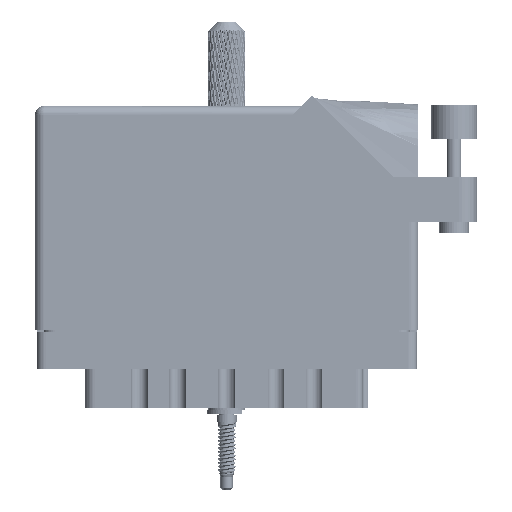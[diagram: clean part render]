
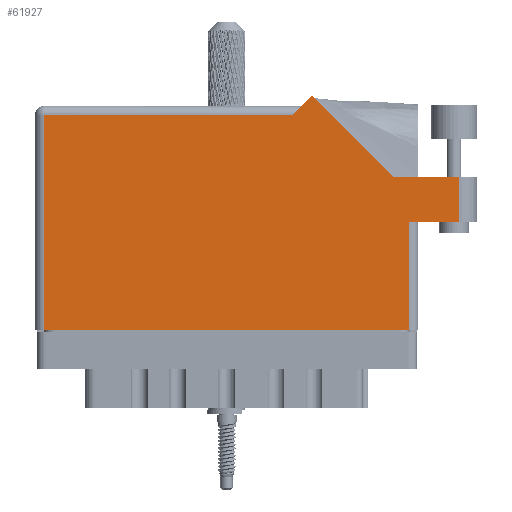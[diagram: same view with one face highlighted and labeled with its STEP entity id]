
A CAD part, front view. The second image highlights one B-rep face of the part: STEP entity #61927.
In plain terms, the highlighted face is planar.
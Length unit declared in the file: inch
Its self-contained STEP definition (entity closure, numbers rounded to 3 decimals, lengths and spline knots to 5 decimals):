
#148 = DIRECTION ( 'NONE',  ( -0.707, -0.707, 0. ) ) ;
#221 = CARTESIAN_POINT ( 'NONE',  ( 2.612, 0.737, 0. ) ) ;
#1091 = VECTOR ( 'NONE', #113292, 39.37008 ) ;
#3236 = ORIENTED_EDGE ( 'NONE', *, *, #10698, .T. ) ;
#4118 = CARTESIAN_POINT ( 'NONE',  ( 3.012, 1.044, 0. ) ) ;
#5088 = PLANE ( 'NONE',  #23254 ) ;
#5506 = CARTESIAN_POINT ( 'NONE',  ( 2.55, 0.737, 0. ) ) ;
#5569 = ORIENTED_EDGE ( 'NONE', *, *, #105520, .T. ) ;
#5610 = VECTOR ( 'NONE', #78746, 39.37008 ) ;
#6254 = ORIENTED_EDGE ( 'NONE', *, *, #28979, .T. ) ;
#9089 = ORIENTED_EDGE ( 'NONE', *, *, #114482, .T. ) ;
#10331 = VERTEX_POINT ( 'NONE', #107970 ) ;
#10432 = EDGE_CURVE ( 'NONE', #11539, #47254, #103604, .T. ) ;
#10698 = EDGE_CURVE ( 'NONE', #10331, #19697, #19981, .T. ) ;
#11539 = VERTEX_POINT ( 'NONE', #89694 ) ;
#16987 = CARTESIAN_POINT ( 'NONE',  ( 0.062, 1.468, 0. ) ) ;
#18177 = CARTESIAN_POINT ( 'NONE',  ( 1.88971, 1.60071, 0. ) ) ;
#19497 = CARTESIAN_POINT ( 'NONE',  ( 2.887, 1.044, 0. ) ) ;
#19697 = VERTEX_POINT ( 'NONE', #18177 ) ;
#19981 = LINE ( 'NONE', #33918, #57261 ) ;
#20785 = DIRECTION ( 'NONE',  ( 0., 1., 0. ) ) ;
#22708 = ORIENTED_EDGE ( 'NONE', *, *, #89235, .T. ) ;
#23254 = AXIS2_PLACEMENT_3D ( 'NONE', #51756, #69391, #118235 ) ;
#23885 = DIRECTION ( 'NONE',  ( -0.707, 0.707, 0. ) ) ;
#24387 = LINE ( 'NONE', #19497, #94914 ) ;
#24979 = ORIENTED_EDGE ( 'NONE', *, *, #115532, .T. ) ;
#25235 = VECTOR ( 'NONE', #41945, 39.37008 ) ;
#28131 = EDGE_LOOP ( 'NONE', ( #24979, #9089, #22708, #3236, #73229, #102067, #106604, #6254, #5569 ) ) ;
#28979 = EDGE_CURVE ( 'NONE', #78155, #74964, #81233, .T. ) ;
#33918 = CARTESIAN_POINT ( 'NONE',  ( 2.44642, 1.044, 0. ) ) ;
#35378 = DIRECTION ( 'NONE',  ( 0., -1., 0. ) ) ;
#35603 = CARTESIAN_POINT ( 'NONE',  ( 1.819, 1.53, 0. ) ) ;
#41945 = DIRECTION ( 'NONE',  ( -1., 0., 0. ) ) ;
#43129 = VERTEX_POINT ( 'NONE', #89583 ) ;
#47254 = VERTEX_POINT ( 'NONE', #16987 ) ;
#47324 = CARTESIAN_POINT ( 'NONE',  ( 2.55, 0.737, 0. ) ) ;
#49379 = CARTESIAN_POINT ( 'NONE',  ( 0., 1.468, 0. ) ) ;
#49809 = CARTESIAN_POINT ( 'NONE',  ( 0., 0., 0. ) ) ;
#51756 = CARTESIAN_POINT ( 'NONE',  ( 0., 1.53, 0. ) ) ;
#54498 = VECTOR ( 'NONE', #35378, 39.37008 ) ;
#56486 = LINE ( 'NONE', #47324, #67952 ) ;
#57261 = VECTOR ( 'NONE', #23885, 39.37008 ) ;
#59903 = VERTEX_POINT ( 'NONE', #5506 ) ;
#61114 = LINE ( 'NONE', #35603, #95768 ) ;
#61927 = ADVANCED_FACE ( 'NONE', ( #89214 ), #5088, .F. ) ;
#67807 = DIRECTION ( 'NONE',  ( 1., 0., 0. ) ) ;
#67952 = VECTOR ( 'NONE', #20785, 39.37008 ) ;
#69391 = DIRECTION ( 'NONE',  ( 0., 0., -1. ) ) ;
#70201 = EDGE_CURVE ( 'NONE', #47254, #78155, #79018, .T. ) ;
#73229 = ORIENTED_EDGE ( 'NONE', *, *, #113468, .T. ) ;
#74438 = LINE ( 'NONE', #221, #1091 ) ;
#74964 = VERTEX_POINT ( 'NONE', #119084 ) ;
#78155 = VERTEX_POINT ( 'NONE', #96973 ) ;
#78746 = DIRECTION ( 'NONE',  ( -1., 0., 0. ) ) ;
#79018 = LINE ( 'NONE', #99855, #54498 ) ;
#81233 = LINE ( 'NONE', #49809, #91260 ) ;
#87028 = LINE ( 'NONE', #4118, #25235 ) ;
#89214 = FACE_OUTER_BOUND ( 'NONE', #28131, .T. ) ;
#89235 = EDGE_CURVE ( 'NONE', #104139, #10331, #87028, .T. ) ;
#89583 = CARTESIAN_POINT ( 'NONE',  ( 2.887, 0.737, 0. ) ) ;
#89694 = CARTESIAN_POINT ( 'NONE',  ( 1.757, 1.468, 0. ) ) ;
#91260 = VECTOR ( 'NONE', #67807, 39.37008 ) ;
#94914 = VECTOR ( 'NONE', #110900, 39.37008 ) ;
#95768 = VECTOR ( 'NONE', #148, 39.37008 ) ;
#96243 = CARTESIAN_POINT ( 'NONE',  ( 2.887, 1.044, 0. ) ) ;
#96973 = CARTESIAN_POINT ( 'NONE',  ( 0.062, 0., 0. ) ) ;
#99855 = CARTESIAN_POINT ( 'NONE',  ( 0.062, 0., 0. ) ) ;
#102067 = ORIENTED_EDGE ( 'NONE', *, *, #10432, .T. ) ;
#103604 = LINE ( 'NONE', #49379, #5610 ) ;
#104139 = VERTEX_POINT ( 'NONE', #96243 ) ;
#105520 = EDGE_CURVE ( 'NONE', #74964, #59903, #56486, .T. ) ;
#106604 = ORIENTED_EDGE ( 'NONE', *, *, #70201, .T. ) ;
#107970 = CARTESIAN_POINT ( 'NONE',  ( 2.44642, 1.044, 0. ) ) ;
#110900 = DIRECTION ( 'NONE',  ( 0., 1., 0. ) ) ;
#113292 = DIRECTION ( 'NONE',  ( 1., 0., 0. ) ) ;
#113468 = EDGE_CURVE ( 'NONE', #19697, #11539, #61114, .T. ) ;
#114482 = EDGE_CURVE ( 'NONE', #43129, #104139, #24387, .T. ) ;
#115532 = EDGE_CURVE ( 'NONE', #59903, #43129, #74438, .T. ) ;
#118235 = DIRECTION ( 'NONE',  ( -1., 0., 0. ) ) ;
#119084 = CARTESIAN_POINT ( 'NONE',  ( 2.55, 0., 0. ) ) ;
